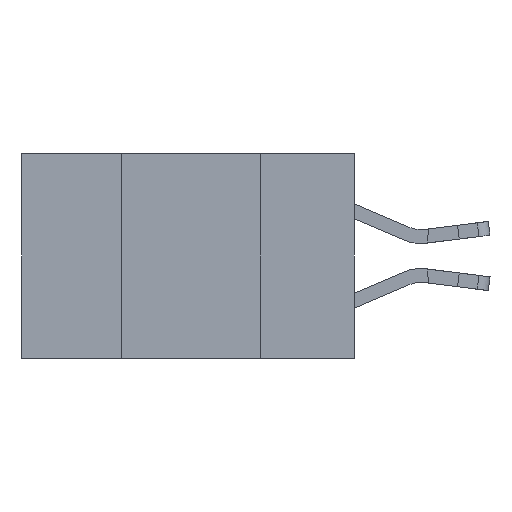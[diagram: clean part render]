
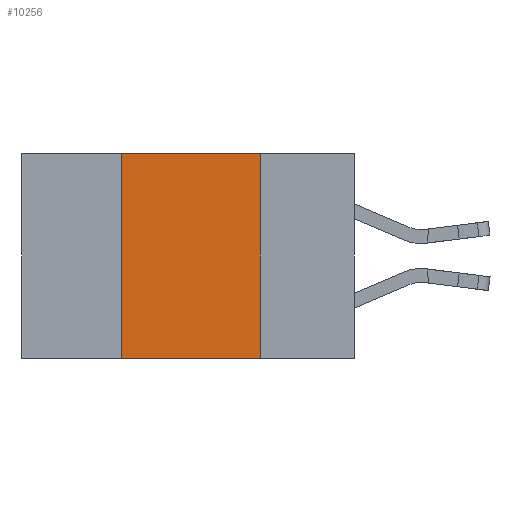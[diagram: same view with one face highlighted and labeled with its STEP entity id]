
A CAD part, left-side view. The second image highlights one B-rep face of the part: STEP entity #10256.
In plain terms, the highlighted planar face has unit normal (-1, 0, 0).
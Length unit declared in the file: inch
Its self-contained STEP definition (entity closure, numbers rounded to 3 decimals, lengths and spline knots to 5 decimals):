
#193 = DIRECTION ( 'NONE',  ( 0., 0., -1. ) ) ;
#273 = DIRECTION ( 'NONE',  ( 1., 0., 0. ) ) ;
#878 = DIRECTION ( 'NONE',  ( 0., -1., 0. ) ) ;
#1154 = VECTOR ( 'NONE', #16654, 39.37008 ) ;
#2671 = CARTESIAN_POINT ( 'NONE',  ( 0., 0.17, 0. ) ) ;
#2744 = VERTEX_POINT ( 'NONE', #4412 ) ;
#3249 = VECTOR ( 'NONE', #11579, 39.37008 ) ;
#3779 = CARTESIAN_POINT ( 'NONE',  ( 0., 0.17, 0. ) ) ;
#3974 = CARTESIAN_POINT ( 'NONE',  ( 0., 0.42, -0.37 ) ) ;
#4336 = LINE ( 'NONE', #21281, #22247 ) ;
#4412 = CARTESIAN_POINT ( 'NONE',  ( 0., 0.17, -0.37 ) ) ;
#5977 = ORIENTED_EDGE ( 'NONE', *, *, #18153, .F. ) ;
#6739 = CARTESIAN_POINT ( 'NONE',  ( 0., 0.6, 0. ) ) ;
#6806 = ORIENTED_EDGE ( 'NONE', *, *, #7764, .T. ) ;
#7764 = EDGE_CURVE ( 'NONE', #18125, #2744, #18649, .T. ) ;
#8626 = VECTOR ( 'NONE', #878, 39.37008 ) ;
#10059 = CARTESIAN_POINT ( 'NONE',  ( 0., 0.6, 0. ) ) ;
#10256 = ADVANCED_FACE ( 'NONE', ( #22876 ), #19493, .F. ) ;
#11190 = LINE ( 'NONE', #6739, #1154 ) ;
#11579 = DIRECTION ( 'NONE',  ( 0., 0., -1. ) ) ;
#11726 = AXIS2_PLACEMENT_3D ( 'NONE', #10059, #273, #193 ) ;
#13106 = ORIENTED_EDGE ( 'NONE', *, *, #19947, .F. ) ;
#13292 = VERTEX_POINT ( 'NONE', #14255 ) ;
#13868 = VERTEX_POINT ( 'NONE', #2671 ) ;
#13983 = EDGE_LOOP ( 'NONE', ( #13106, #5977, #14986, #6806 ) ) ;
#14255 = CARTESIAN_POINT ( 'NONE',  ( 0., 0.42, 0. ) ) ;
#14986 = ORIENTED_EDGE ( 'NONE', *, *, #22826, .F. ) ;
#16654 = DIRECTION ( 'NONE',  ( 0., -1., 0. ) ) ;
#17706 = DIRECTION ( 'NONE',  ( 0., 0., 1. ) ) ;
#18125 = VERTEX_POINT ( 'NONE', #3974 ) ;
#18153 = EDGE_CURVE ( 'NONE', #13292, #13868, #11190, .T. ) ;
#18649 = LINE ( 'NONE', #20439, #8626 ) ;
#19493 = PLANE ( 'NONE',  #11726 ) ;
#19947 = EDGE_CURVE ( 'NONE', #13868, #2744, #20871, .T. ) ;
#20439 = CARTESIAN_POINT ( 'NONE',  ( 0., 0.6, -0.37 ) ) ;
#20871 = LINE ( 'NONE', #3779, #3249 ) ;
#21281 = CARTESIAN_POINT ( 'NONE',  ( 0., 0.42, 0. ) ) ;
#22247 = VECTOR ( 'NONE', #17706, 39.37008 ) ;
#22826 = EDGE_CURVE ( 'NONE', #18125, #13292, #4336, .T. ) ;
#22876 = FACE_OUTER_BOUND ( 'NONE', #13983, .T. ) ;
